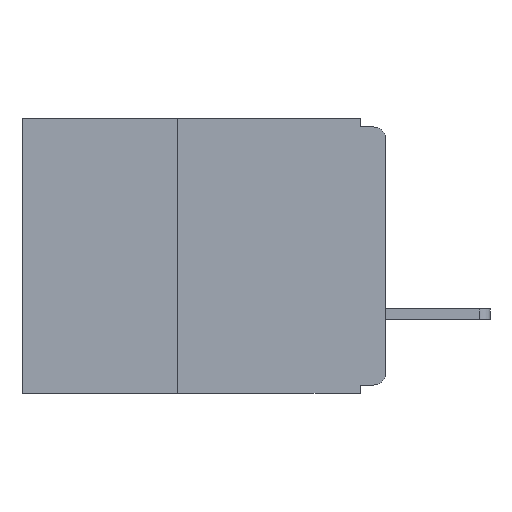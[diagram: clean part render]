
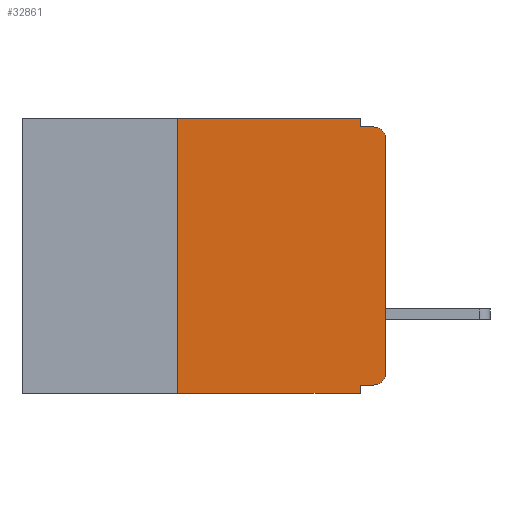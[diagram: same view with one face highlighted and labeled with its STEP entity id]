
A CAD part, left-side view. The second image highlights one B-rep face of the part: STEP entity #32861.
In plain terms, the highlighted planar face has unit normal (-1, 0, 0).
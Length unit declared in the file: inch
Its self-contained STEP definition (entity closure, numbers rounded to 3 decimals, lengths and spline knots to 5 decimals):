
#50 = EDGE_CURVE ( 'NONE', #9942, #8943, #30408, .T. ) ;
#545 = LINE ( 'NONE', #13308, #14252 ) ;
#661 = CIRCLE ( 'NONE', #34599, 0.015 ) ;
#952 = CARTESIAN_POINT ( 'NONE',  ( 0., 0.031, -0.01 ) ) ;
#1603 = CARTESIAN_POINT ( 'NONE',  ( 0., 0.031, -0.33 ) ) ;
#1953 = CARTESIAN_POINT ( 'NONE',  ( 0., 0.25, -0.33 ) ) ;
#2161 = ORIENTED_EDGE ( 'NONE', *, *, #33857, .F. ) ;
#2740 = CARTESIAN_POINT ( 'NONE',  ( 0., 0.25, -0.33 ) ) ;
#4214 = VERTEX_POINT ( 'NONE', #952 ) ;
#4282 = VERTEX_POINT ( 'NONE', #9511 ) ;
#4330 = LINE ( 'NONE', #1953, #10762 ) ;
#4481 = ORIENTED_EDGE ( 'NONE', *, *, #19091, .F. ) ;
#5009 = VERTEX_POINT ( 'NONE', #26066 ) ;
#5899 = DIRECTION ( 'NONE',  ( 0., -1., 0. ) ) ;
#5960 = EDGE_CURVE ( 'NONE', #19307, #5009, #545, .T. ) ;
#6047 = VECTOR ( 'NONE', #14410, 39.37008 ) ;
#6489 = ORIENTED_EDGE ( 'NONE', *, *, #50, .F. ) ;
#6497 = CIRCLE ( 'NONE', #30024, 0.015 ) ;
#7061 = CARTESIAN_POINT ( 'NONE',  ( 0., 0., -0.32 ) ) ;
#8432 = CARTESIAN_POINT ( 'NONE',  ( 0., 0.015, -0.025 ) ) ;
#8497 = VERTEX_POINT ( 'NONE', #2740 ) ;
#8943 = VERTEX_POINT ( 'NONE', #1603 ) ;
#8959 = DIRECTION ( 'NONE',  ( 0., 0., -1. ) ) ;
#9511 = CARTESIAN_POINT ( 'NONE',  ( 0., 0.031, 0. ) ) ;
#9797 = DIRECTION ( 'NONE',  ( 0., 1., 0. ) ) ;
#9942 = VERTEX_POINT ( 'NONE', #32938 ) ;
#10510 = ORIENTED_EDGE ( 'NONE', *, *, #5960, .T. ) ;
#10589 = DIRECTION ( 'NONE',  ( 0., 0., -1. ) ) ;
#10609 = DIRECTION ( 'NONE',  ( 0., 0., 1. ) ) ;
#10762 = VECTOR ( 'NONE', #23822, 39.37008 ) ;
#11153 = DIRECTION ( 'NONE',  ( 0., 0., -1. ) ) ;
#11712 = CARTESIAN_POINT ( 'NONE',  ( 0., 0.015, -0.01 ) ) ;
#11738 = EDGE_LOOP ( 'NONE', ( #10510, #15074, #11899, #23730, #4481, #26391, #15930, #6489, #2161, #18707 ) ) ;
#11899 = ORIENTED_EDGE ( 'NONE', *, *, #15502, .F. ) ;
#12934 = VERTEX_POINT ( 'NONE', #24633 ) ;
#13308 = CARTESIAN_POINT ( 'NONE',  ( 0., 0., 0. ) ) ;
#13473 = DIRECTION ( 'NONE',  ( -1., 0., 0. ) ) ;
#13493 = CARTESIAN_POINT ( 'NONE',  ( 0., 0.031, -0.33 ) ) ;
#14252 = VECTOR ( 'NONE', #10609, 39.37008 ) ;
#14297 = CARTESIAN_POINT ( 'NONE',  ( 0., 0., -0.305 ) ) ;
#14410 = DIRECTION ( 'NONE',  ( 0., -1., 0. ) ) ;
#15074 = ORIENTED_EDGE ( 'NONE', *, *, #23758, .T. ) ;
#15288 = EDGE_CURVE ( 'NONE', #12934, #19307, #6497, .T. ) ;
#15502 = EDGE_CURVE ( 'NONE', #4214, #29301, #27592, .T. ) ;
#15930 = ORIENTED_EDGE ( 'NONE', *, *, #18610, .T. ) ;
#16089 = DIRECTION ( 'NONE',  ( 0., -1., 0. ) ) ;
#16143 = VECTOR ( 'NONE', #10589, 39.37008 ) ;
#16149 = DIRECTION ( 'NONE',  ( 0., 0., -1. ) ) ;
#17575 = EDGE_CURVE ( 'NONE', #4282, #4214, #19045, .T. ) ;
#18610 = EDGE_CURVE ( 'NONE', #8497, #8943, #19018, .T. ) ;
#18707 = ORIENTED_EDGE ( 'NONE', *, *, #15288, .T. ) ;
#19018 = LINE ( 'NONE', #30075, #25269 ) ;
#19045 = LINE ( 'NONE', #27809, #24464 ) ;
#19091 = EDGE_CURVE ( 'NONE', #28479, #4282, #24408, .T. ) ;
#19307 = VERTEX_POINT ( 'NONE', #14297 ) ;
#21919 = FACE_OUTER_BOUND ( 'NONE', #11738, .T. ) ;
#22257 = VECTOR ( 'NONE', #9797, 39.37008 ) ;
#23573 = VECTOR ( 'NONE', #16089, 39.37008 ) ;
#23730 = ORIENTED_EDGE ( 'NONE', *, *, #17575, .F. ) ;
#23758 = EDGE_CURVE ( 'NONE', #5009, #29301, #661, .T. ) ;
#23822 = DIRECTION ( 'NONE',  ( 0., 0., 1. ) ) ;
#23923 = LINE ( 'NONE', #7061, #22257 ) ;
#24135 = CARTESIAN_POINT ( 'NONE',  ( 0., 0.437, 0. ) ) ;
#24408 = LINE ( 'NONE', #34727, #23573 ) ;
#24464 = VECTOR ( 'NONE', #8959, 39.37008 ) ;
#24633 = CARTESIAN_POINT ( 'NONE',  ( 0., 0.015, -0.32 ) ) ;
#25269 = VECTOR ( 'NONE', #5899, 39.37008 ) ;
#26066 = CARTESIAN_POINT ( 'NONE',  ( 0., 0., -0.025 ) ) ;
#26391 = ORIENTED_EDGE ( 'NONE', *, *, #28361, .F. ) ;
#27277 = DIRECTION ( 'NONE',  ( -1., 0., 0. ) ) ;
#27592 = LINE ( 'NONE', #33125, #6047 ) ;
#27809 = CARTESIAN_POINT ( 'NONE',  ( 0., 0.031, 0. ) ) ;
#28361 = EDGE_CURVE ( 'NONE', #8497, #28479, #4330, .T. ) ;
#28479 = VERTEX_POINT ( 'NONE', #34932 ) ;
#29301 = VERTEX_POINT ( 'NONE', #11712 ) ;
#29501 = PLANE ( 'NONE',  #32975 ) ;
#29568 = CARTESIAN_POINT ( 'NONE',  ( 0., 0.015, -0.305 ) ) ;
#30024 = AXIS2_PLACEMENT_3D ( 'NONE', #29568, #13473, #32218 ) ;
#30075 = CARTESIAN_POINT ( 'NONE',  ( 0., 0.437, -0.33 ) ) ;
#30408 = LINE ( 'NONE', #13493, #16143 ) ;
#32151 = DIRECTION ( 'NONE',  ( 1., 0., 0. ) ) ;
#32218 = DIRECTION ( 'NONE',  ( 0., 0., -1. ) ) ;
#32861 = ADVANCED_FACE ( 'NONE', ( #21919 ), #29501, .F. ) ;
#32938 = CARTESIAN_POINT ( 'NONE',  ( 0., 0.031, -0.32 ) ) ;
#32975 = AXIS2_PLACEMENT_3D ( 'NONE', #24135, #32151, #16149 ) ;
#33125 = CARTESIAN_POINT ( 'NONE',  ( 0., 0., -0.01 ) ) ;
#33857 = EDGE_CURVE ( 'NONE', #12934, #9942, #23923, .T. ) ;
#34599 = AXIS2_PLACEMENT_3D ( 'NONE', #8432, #27277, #11153 ) ;
#34727 = CARTESIAN_POINT ( 'NONE',  ( 0., 0.437, 0. ) ) ;
#34932 = CARTESIAN_POINT ( 'NONE',  ( 0., 0.25, 0. ) ) ;
